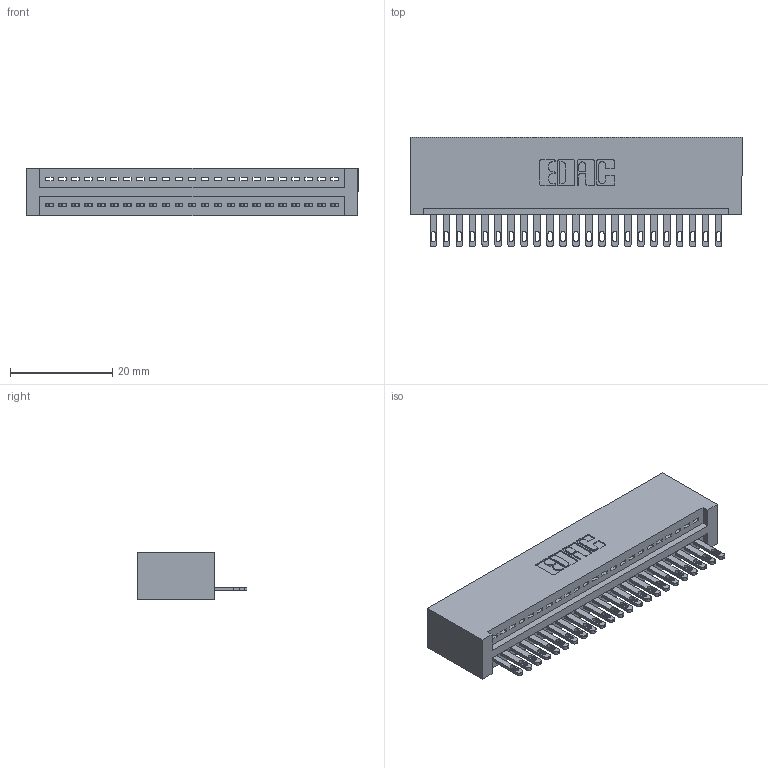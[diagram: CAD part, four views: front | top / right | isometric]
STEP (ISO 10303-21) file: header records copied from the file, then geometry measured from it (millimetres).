
FILE_DESCRIPTION (( 'STEP AP203' ), '1' );
FILE_NAME ('345-023-500-101.STEP', '2019-10-05T01:17:07', ( '' ), ( '' ), 'SwSTEP 2.0', 'SolidWorks 2016', '' );
FILE_SCHEMA (( 'CONFIG_CONTROL_DESIGN' ));
Length unit declared in the file: inch
Products named in the file (3): 345-292-001_345-293-100; 345 Part_No Mounting Lugs; 345-023-500-101
Assembly tree (24 placements, depth 2):
  345-023-500-101
    345 Part_No Mounting Lugs
    345-292-001_345-293-100  x23
Bounding box: 65.02 x 21.51 x 9.4 mm (x, y, z)
Volume: 6619 mm3; surface area: 8779.6 mm2
Topology: 24 solids, 24 shells, 1360 faces, 4181 edges, 2786 vertices
Faces by surface type: plane 858, cylinder 502
Entity records: 19521 total; most frequent: CARTESIAN_POINT 3389, ORIENTED_EDGE 3346, DIRECTION 2983, EDGE_CURVE 1673, LINE 1453, VECTOR 1453, VERTEX_POINT 1114, AXIS2_PLACEMENT_3D 765
